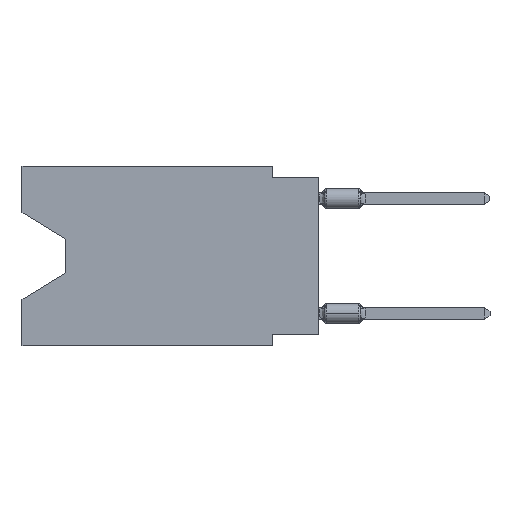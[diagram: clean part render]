
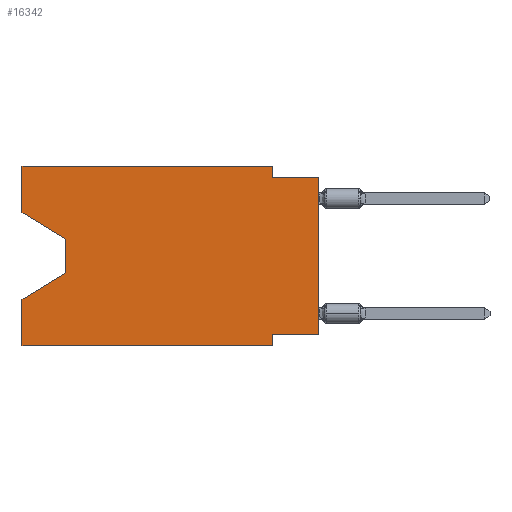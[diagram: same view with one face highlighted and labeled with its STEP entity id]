
A CAD part, left-side view. The second image highlights one B-rep face of the part: STEP entity #16342.
In plain terms, the highlighted planar face has unit normal (-1, 0, 0).
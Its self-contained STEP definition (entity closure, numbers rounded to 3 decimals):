
#174 = FACE_OUTER_BOUND ( 'NONE', #6839, .T. ) ;
#301 = VERTEX_POINT ( 'NONE', #7257 ) ;
#358 = CARTESIAN_POINT ( 'NONE',  ( 0., 13.97, -5.893 ) ) ;
#418 = DIRECTION ( 'NONE',  ( 0., 0., 1. ) ) ;
#673 = VECTOR ( 'NONE', #12801, 1000. ) ;
#740 = EDGE_CURVE ( 'NONE', #15916, #2981, #6068, .T. ) ;
#870 = CARTESIAN_POINT ( 'NONE',  ( 0., 0., -9.271 ) ) ;
#937 = LINE ( 'NONE', #15273, #7613 ) ;
#974 = CARTESIAN_POINT ( 'NONE',  ( 0., 13.97, -4.013 ) ) ;
#1099 = CARTESIAN_POINT ( 'NONE',  ( 0., 16.383, -2.546 ) ) ;
#1228 = EDGE_CURVE ( 'NONE', #14280, #14696, #15095, .T. ) ;
#1276 = DIRECTION ( 'NONE',  ( 0., 0.855, -0.519 ) ) ;
#1378 = ORIENTED_EDGE ( 'NONE', *, *, #8464, .T. ) ;
#1603 = ORIENTED_EDGE ( 'NONE', *, *, #16942, .F. ) ;
#1620 = DIRECTION ( 'NONE',  ( 0., -1., 0. ) ) ;
#1858 = EDGE_CURVE ( 'NONE', #5714, #14447, #9349, .T. ) ;
#1978 = DIRECTION ( 'NONE',  ( 0., 0., -1. ) ) ;
#2381 = VERTEX_POINT ( 'NONE', #15652 ) ;
#2389 = CARTESIAN_POINT ( 'NONE',  ( 0., 0., -0.635 ) ) ;
#2641 = EDGE_CURVE ( 'NONE', #14280, #2381, #4055, .T. ) ;
#2724 = CARTESIAN_POINT ( 'NONE',  ( 0., 13.97, -4.013 ) ) ;
#2922 = ORIENTED_EDGE ( 'NONE', *, *, #13971, .F. ) ;
#2981 = VERTEX_POINT ( 'NONE', #12434 ) ;
#3080 = LINE ( 'NONE', #4467, #15869 ) ;
#3214 = DIRECTION ( 'NONE',  ( 0., 1., 0. ) ) ;
#3281 = DIRECTION ( 'NONE',  ( 0., 0., 1. ) ) ;
#3552 = CARTESIAN_POINT ( 'NONE',  ( 0., 16.383, 0. ) ) ;
#4055 = LINE ( 'NONE', #8063, #5630 ) ;
#4467 = CARTESIAN_POINT ( 'NONE',  ( 0., 16.383, 0. ) ) ;
#4754 = DIRECTION ( 'NONE',  ( 0., 0., -1. ) ) ;
#4909 = CARTESIAN_POINT ( 'NONE',  ( 0., 13.97, -5.893 ) ) ;
#5162 = DIRECTION ( 'NONE',  ( 0., 0., -1. ) ) ;
#5223 = LINE ( 'NONE', #974, #15421 ) ;
#5539 = CARTESIAN_POINT ( 'NONE',  ( 0., 16.383, 0. ) ) ;
#5630 = VECTOR ( 'NONE', #1620, 1000. ) ;
#5714 = VERTEX_POINT ( 'NONE', #16259 ) ;
#6063 = LINE ( 'NONE', #3552, #7984 ) ;
#6068 = LINE ( 'NONE', #13723, #13419 ) ;
#6300 = LINE ( 'NONE', #2389, #673 ) ;
#6444 = VERTEX_POINT ( 'NONE', #2724 ) ;
#6678 = EDGE_CURVE ( 'NONE', #6444, #17022, #5223, .T. ) ;
#6839 = EDGE_LOOP ( 'NONE', ( #1378, #15881, #10265, #13099, #11204, #2922, #16952, #9779, #8207, #12253, #1603, #12690 ) ) ;
#6877 = PLANE ( 'NONE',  #15568 ) ;
#7226 = CARTESIAN_POINT ( 'NONE',  ( 0., 16.383, -7.36 ) ) ;
#7257 = CARTESIAN_POINT ( 'NONE',  ( 0., 16.383, 0. ) ) ;
#7613 = VECTOR ( 'NONE', #1978, 1000. ) ;
#7984 = VECTOR ( 'NONE', #8860, 1000. ) ;
#8055 = LINE ( 'NONE', #358, #15471 ) ;
#8063 = CARTESIAN_POINT ( 'NONE',  ( 0., 16.383, -9.906 ) ) ;
#8207 = ORIENTED_EDGE ( 'NONE', *, *, #11557, .F. ) ;
#8262 = EDGE_CURVE ( 'NONE', #8679, #301, #6063, .T. ) ;
#8464 = EDGE_CURVE ( 'NONE', #8679, #6444, #13613, .T. ) ;
#8679 = VERTEX_POINT ( 'NONE', #1099 ) ;
#8836 = EDGE_CURVE ( 'NONE', #17022, #14696, #8055, .T. ) ;
#8860 = DIRECTION ( 'NONE',  ( 0., 0., 1. ) ) ;
#9349 = LINE ( 'NONE', #17081, #9560 ) ;
#9482 = CARTESIAN_POINT ( 'NONE',  ( 0., 2.54, -0.635 ) ) ;
#9560 = VECTOR ( 'NONE', #5162, 1000. ) ;
#9778 = DIRECTION ( 'NONE',  ( 0., -1., 0. ) ) ;
#9779 = ORIENTED_EDGE ( 'NONE', *, *, #10964, .T. ) ;
#10048 = CARTESIAN_POINT ( 'NONE',  ( 0., 0., 0. ) ) ;
#10142 = CARTESIAN_POINT ( 'NONE',  ( 0., 0., -0.635 ) ) ;
#10265 = ORIENTED_EDGE ( 'NONE', *, *, #8836, .T. ) ;
#10643 = VECTOR ( 'NONE', #3281, 1000. ) ;
#10964 = EDGE_CURVE ( 'NONE', #15916, #12351, #12561, .T. ) ;
#10974 = CARTESIAN_POINT ( 'NONE',  ( 0., 16.383, -9.906 ) ) ;
#11204 = ORIENTED_EDGE ( 'NONE', *, *, #2641, .T. ) ;
#11557 = EDGE_CURVE ( 'NONE', #14447, #12351, #6300, .T. ) ;
#12253 = ORIENTED_EDGE ( 'NONE', *, *, #1858, .F. ) ;
#12351 = VERTEX_POINT ( 'NONE', #10142 ) ;
#12434 = CARTESIAN_POINT ( 'NONE',  ( 0., 2.54, -9.271 ) ) ;
#12561 = LINE ( 'NONE', #10048, #16251 ) ;
#12690 = ORIENTED_EDGE ( 'NONE', *, *, #8262, .F. ) ;
#12801 = DIRECTION ( 'NONE',  ( 0., -1., 0. ) ) ;
#12964 = DIRECTION ( 'NONE',  ( 0., 0., -1. ) ) ;
#13099 = ORIENTED_EDGE ( 'NONE', *, *, #1228, .F. ) ;
#13419 = VECTOR ( 'NONE', #3214, 1000. ) ;
#13453 = CARTESIAN_POINT ( 'NONE',  ( 0., 16.383, -2.546 ) ) ;
#13535 = DIRECTION ( 'NONE',  ( 0., -0.855, -0.519 ) ) ;
#13613 = LINE ( 'NONE', #13453, #16859 ) ;
#13723 = CARTESIAN_POINT ( 'NONE',  ( 0., 0., -9.271 ) ) ;
#13971 = EDGE_CURVE ( 'NONE', #2981, #2381, #937, .T. ) ;
#14280 = VERTEX_POINT ( 'NONE', #10974 ) ;
#14447 = VERTEX_POINT ( 'NONE', #9482 ) ;
#14696 = VERTEX_POINT ( 'NONE', #7226 ) ;
#14854 = DIRECTION ( 'NONE',  ( 1., 0., 0. ) ) ;
#14930 = CARTESIAN_POINT ( 'NONE',  ( 0., 16.383, 0. ) ) ;
#15095 = LINE ( 'NONE', #14930, #10643 ) ;
#15273 = CARTESIAN_POINT ( 'NONE',  ( 0., 2.54, -9.906 ) ) ;
#15421 = VECTOR ( 'NONE', #12964, 1000. ) ;
#15471 = VECTOR ( 'NONE', #1276, 1000. ) ;
#15568 = AXIS2_PLACEMENT_3D ( 'NONE', #5539, #14854, #4754 ) ;
#15652 = CARTESIAN_POINT ( 'NONE',  ( 0., 2.54, -9.906 ) ) ;
#15869 = VECTOR ( 'NONE', #9778, 1000. ) ;
#15881 = ORIENTED_EDGE ( 'NONE', *, *, #6678, .T. ) ;
#15916 = VERTEX_POINT ( 'NONE', #870 ) ;
#16251 = VECTOR ( 'NONE', #418, 1000. ) ;
#16259 = CARTESIAN_POINT ( 'NONE',  ( 0., 2.54, 0. ) ) ;
#16342 = ADVANCED_FACE ( 'NONE', ( #174 ), #6877, .F. ) ;
#16859 = VECTOR ( 'NONE', #13535, 1000. ) ;
#16942 = EDGE_CURVE ( 'NONE', #301, #5714, #3080, .T. ) ;
#16952 = ORIENTED_EDGE ( 'NONE', *, *, #740, .F. ) ;
#17022 = VERTEX_POINT ( 'NONE', #4909 ) ;
#17081 = CARTESIAN_POINT ( 'NONE',  ( 0., 2.54, 0. ) ) ;
